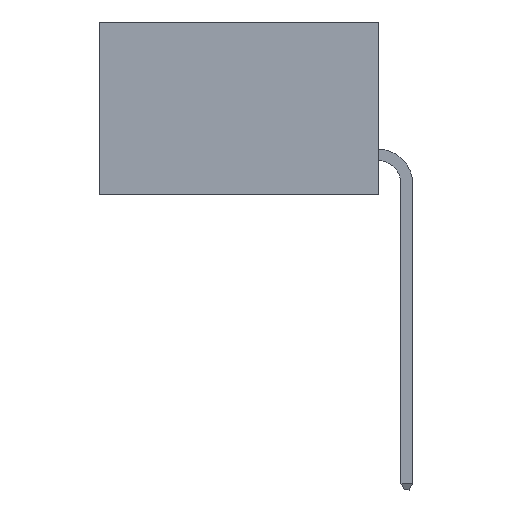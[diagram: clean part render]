
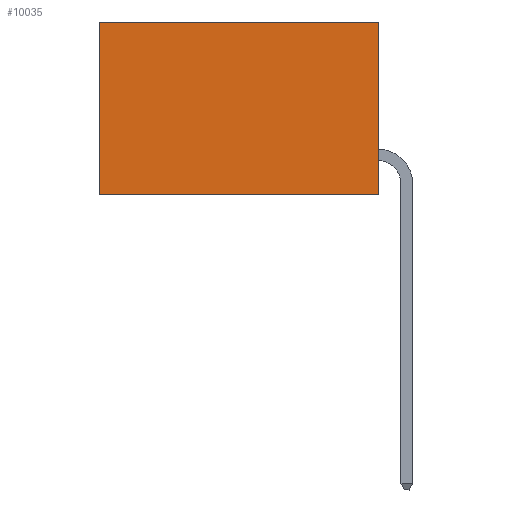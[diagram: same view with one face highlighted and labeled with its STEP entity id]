
A CAD part, left-side view. The second image highlights one B-rep face of the part: STEP entity #10035.
In plain terms, the highlighted planar face has unit normal (-1, 0, 0).
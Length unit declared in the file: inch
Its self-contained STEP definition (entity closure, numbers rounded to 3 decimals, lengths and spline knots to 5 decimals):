
#365 = CARTESIAN_POINT ( 'NONE',  ( 0.298, 0., 0. ) ) ;
#1768 = PLANE ( 'NONE',  #7224 ) ;
#2441 = VERTEX_POINT ( 'NONE', #20434 ) ;
#3949 = FACE_OUTER_BOUND ( 'NONE', #4198, .T. ) ;
#4198 = EDGE_LOOP ( 'NONE', ( #16997, #6549, #12713, #9233 ) ) ;
#4423 = VERTEX_POINT ( 'NONE', #4860 ) ;
#4844 = VECTOR ( 'NONE', #17597, 39.37008 ) ;
#4860 = CARTESIAN_POINT ( 'NONE',  ( 0.298, 0., 0. ) ) ;
#5806 = EDGE_CURVE ( 'NONE', #4423, #20013, #6845, .T. ) ;
#6219 = DIRECTION ( 'NONE',  ( 0., 1., 0. ) ) ;
#6496 = CARTESIAN_POINT ( 'NONE',  ( 0.298, 0., 0. ) ) ;
#6549 = ORIENTED_EDGE ( 'NONE', *, *, #16693, .F. ) ;
#6845 = LINE ( 'NONE', #6496, #4844 ) ;
#7224 = AXIS2_PLACEMENT_3D ( 'NONE', #365, #16145, #11388 ) ;
#8432 = LINE ( 'NONE', #19311, #12182 ) ;
#8587 = EDGE_CURVE ( 'NONE', #4423, #20417, #20369, .T. ) ;
#9233 = ORIENTED_EDGE ( 'NONE', *, *, #5806, .T. ) ;
#10035 = ADVANCED_FACE ( 'NONE', ( #3949 ), #1768, .F. ) ;
#11033 = VECTOR ( 'NONE', #6219, 39.37008 ) ;
#11388 = DIRECTION ( 'NONE',  ( 0., 0., -1. ) ) ;
#12182 = VECTOR ( 'NONE', #14595, 39.37008 ) ;
#12439 = CARTESIAN_POINT ( 'NONE',  ( 0.298, 0.6, 0. ) ) ;
#12713 = ORIENTED_EDGE ( 'NONE', *, *, #8587, .F. ) ;
#13901 = CARTESIAN_POINT ( 'NONE',  ( 0.298, 0., -0.37 ) ) ;
#14595 = DIRECTION ( 'NONE',  ( 0., 0., -1. ) ) ;
#14807 = EDGE_CURVE ( 'NONE', #20013, #2441, #8432, .T. ) ;
#15182 = DIRECTION ( 'NONE',  ( 0., 0., -1. ) ) ;
#15257 = LINE ( 'NONE', #19005, #11033 ) ;
#16145 = DIRECTION ( 'NONE',  ( 1., 0., 0. ) ) ;
#16693 = EDGE_CURVE ( 'NONE', #20417, #2441, #15257, .T. ) ;
#16997 = ORIENTED_EDGE ( 'NONE', *, *, #14807, .T. ) ;
#17597 = DIRECTION ( 'NONE',  ( 0., 1., 0. ) ) ;
#18347 = CARTESIAN_POINT ( 'NONE',  ( 0.298, 0., 0. ) ) ;
#18631 = VECTOR ( 'NONE', #15182, 39.37008 ) ;
#19005 = CARTESIAN_POINT ( 'NONE',  ( 0.298, 0., -0.37 ) ) ;
#19311 = CARTESIAN_POINT ( 'NONE',  ( 0.298, 0.6, 0. ) ) ;
#20013 = VERTEX_POINT ( 'NONE', #12439 ) ;
#20369 = LINE ( 'NONE', #18347, #18631 ) ;
#20417 = VERTEX_POINT ( 'NONE', #13901 ) ;
#20434 = CARTESIAN_POINT ( 'NONE',  ( 0.298, 0.6, -0.37 ) ) ;
